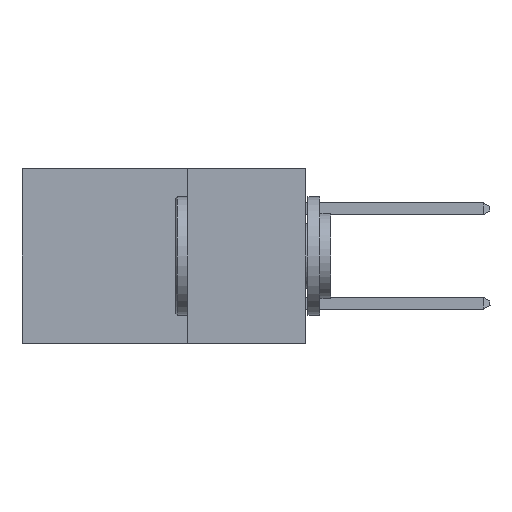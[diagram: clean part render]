
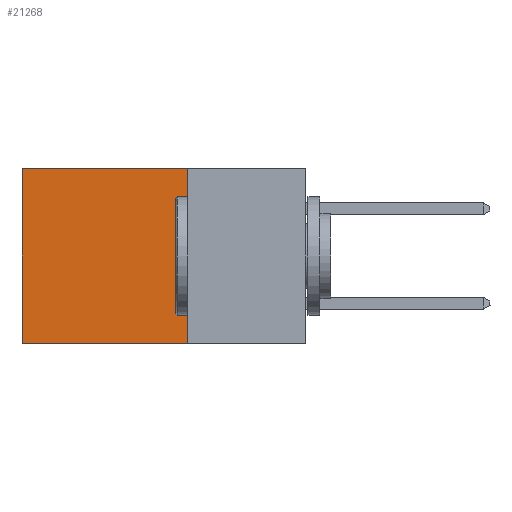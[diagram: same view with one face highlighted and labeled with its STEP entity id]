
A CAD part, left-side view. The second image highlights one B-rep face of the part: STEP entity #21268.
In plain terms, the highlighted planar face has unit normal (-1, 0, 0).
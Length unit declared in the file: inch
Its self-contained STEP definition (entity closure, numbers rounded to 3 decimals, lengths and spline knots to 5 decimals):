
#376 = VECTOR ( 'NONE', #8557, 39.37008 ) ;
#391 = CARTESIAN_POINT ( 'NONE',  ( 0.298, 0.25, 0. ) ) ;
#560 = ORIENTED_EDGE ( 'NONE', *, *, #11187, .F. ) ;
#1833 = EDGE_CURVE ( 'NONE', #11125, #21441, #11619, .T. ) ;
#2190 = CARTESIAN_POINT ( 'NONE',  ( 0.298, 0.25, -0.37 ) ) ;
#2757 = PLANE ( 'NONE',  #23702 ) ;
#5031 = VECTOR ( 'NONE', #20176, 39.37008 ) ;
#5688 = VECTOR ( 'NONE', #10242, 39.37008 ) ;
#7682 = VECTOR ( 'NONE', #11371, 39.37008 ) ;
#8557 = DIRECTION ( 'NONE',  ( 0., 0., -1. ) ) ;
#8633 = EDGE_LOOP ( 'NONE', ( #12231, #11133, #560, #9397 ) ) ;
#8669 = CARTESIAN_POINT ( 'NONE',  ( 0.298, 0.25, 0. ) ) ;
#8922 = DIRECTION ( 'NONE',  ( 1., 0., 0. ) ) ;
#9397 = ORIENTED_EDGE ( 'NONE', *, *, #22693, .T. ) ;
#10217 = CARTESIAN_POINT ( 'NONE',  ( 0.298, 0.25, -0.37 ) ) ;
#10242 = DIRECTION ( 'NONE',  ( 0., 1., 0. ) ) ;
#10462 = CARTESIAN_POINT ( 'NONE',  ( 0.298, 0.25, 0. ) ) ;
#10476 = VERTEX_POINT ( 'NONE', #20030 ) ;
#11125 = VERTEX_POINT ( 'NONE', #2190 ) ;
#11133 = ORIENTED_EDGE ( 'NONE', *, *, #1833, .F. ) ;
#11182 = LINE ( 'NONE', #391, #376 ) ;
#11187 = EDGE_CURVE ( 'NONE', #15313, #11125, #11182, .T. ) ;
#11371 = DIRECTION ( 'NONE',  ( 0., 0., -1. ) ) ;
#11404 = CARTESIAN_POINT ( 'NONE',  ( 0.298, 0.6, -0.37 ) ) ;
#11619 = LINE ( 'NONE', #10217, #5688 ) ;
#12231 = ORIENTED_EDGE ( 'NONE', *, *, #20062, .T. ) ;
#15313 = VERTEX_POINT ( 'NONE', #8669 ) ;
#18131 = FACE_OUTER_BOUND ( 'NONE', #8633, .T. ) ;
#18144 = LINE ( 'NONE', #21095, #7682 ) ;
#20030 = CARTESIAN_POINT ( 'NONE',  ( 0.298, 0.6, 0. ) ) ;
#20062 = EDGE_CURVE ( 'NONE', #10476, #21441, #18144, .T. ) ;
#20176 = DIRECTION ( 'NONE',  ( 0., 1., 0. ) ) ;
#21095 = CARTESIAN_POINT ( 'NONE',  ( 0.298, 0.6, 0. ) ) ;
#21268 = ADVANCED_FACE ( 'NONE', ( #18131 ), #2757, .F. ) ;
#21441 = VERTEX_POINT ( 'NONE', #11404 ) ;
#22533 = DIRECTION ( 'NONE',  ( 0., 0., -1. ) ) ;
#22693 = EDGE_CURVE ( 'NONE', #15313, #10476, #25149, .T. ) ;
#23702 = AXIS2_PLACEMENT_3D ( 'NONE', #24318, #8922, #22533 ) ;
#24318 = CARTESIAN_POINT ( 'NONE',  ( 0.298, 0.25, 0. ) ) ;
#25149 = LINE ( 'NONE', #10462, #5031 ) ;
